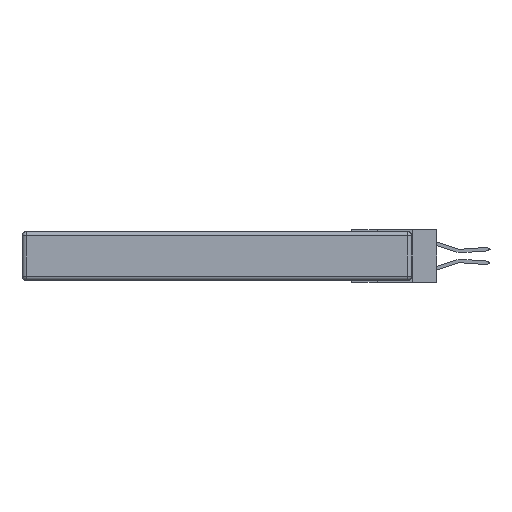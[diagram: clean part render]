
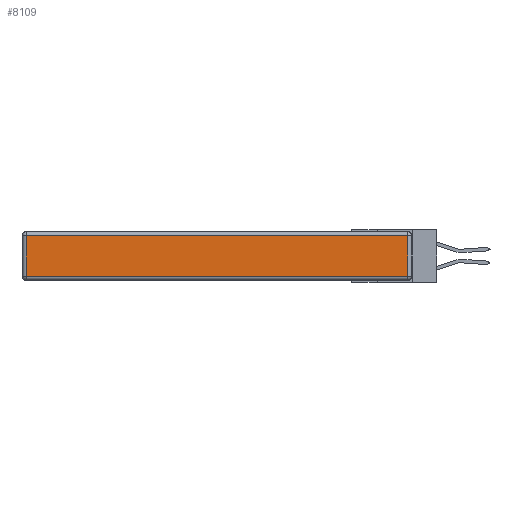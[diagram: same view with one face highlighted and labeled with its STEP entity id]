
A CAD part, left-side view. The second image highlights one B-rep face of the part: STEP entity #8109.
In plain terms, the highlighted planar face has unit normal (-1, 0, 0).
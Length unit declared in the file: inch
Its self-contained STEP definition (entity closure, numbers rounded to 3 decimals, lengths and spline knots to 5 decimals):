
#1151 = VECTOR ( 'NONE', #12823, 39.37008 ) ;
#1198 = DIRECTION ( 'NONE',  ( 0., 0., 1. ) ) ;
#1743 = VECTOR ( 'NONE', #9627, 39.37008 ) ;
#3350 = LINE ( 'NONE', #12667, #1151 ) ;
#3606 = ORIENTED_EDGE ( 'NONE', *, *, #10791, .T. ) ;
#4678 = CARTESIAN_POINT ( 'NONE',  ( 0., 0.03, -0.03 ) ) ;
#4986 = ORIENTED_EDGE ( 'NONE', *, *, #15212, .T. ) ;
#5455 = AXIS2_PLACEMENT_3D ( 'NONE', #11629, #15234, #1198 ) ;
#5585 = CARTESIAN_POINT ( 'NONE',  ( 0., 2.72, -0.03 ) ) ;
#5778 = CARTESIAN_POINT ( 'NONE',  ( 0., 2.72, -0.343 ) ) ;
#5894 = VERTEX_POINT ( 'NONE', #5585 ) ;
#6389 = LINE ( 'NONE', #20187, #1743 ) ;
#7204 = LINE ( 'NONE', #5778, #14309 ) ;
#7402 = VERTEX_POINT ( 'NONE', #13317 ) ;
#8109 = ADVANCED_FACE ( 'NONE', ( #10407 ), #11555, .T. ) ;
#9242 = DIRECTION ( 'NONE',  ( 0., 0., 1. ) ) ;
#9627 = DIRECTION ( 'NONE',  ( 0., -1., 0. ) ) ;
#9665 = EDGE_CURVE ( 'NONE', #5894, #7402, #7204, .T. ) ;
#10407 = FACE_OUTER_BOUND ( 'NONE', #15792, .T. ) ;
#10791 = EDGE_CURVE ( 'NONE', #18504, #5894, #3350, .T. ) ;
#11555 = PLANE ( 'NONE',  #5455 ) ;
#11617 = VERTEX_POINT ( 'NONE', #22510 ) ;
#11629 = CARTESIAN_POINT ( 'NONE',  ( 0., 0., -0.343 ) ) ;
#12127 = VECTOR ( 'NONE', #9242, 39.37008 ) ;
#12667 = CARTESIAN_POINT ( 'NONE',  ( 0., 2.75, -0.03 ) ) ;
#12823 = DIRECTION ( 'NONE',  ( 0., 1., 0. ) ) ;
#13317 = CARTESIAN_POINT ( 'NONE',  ( 0., 2.72, -0.313 ) ) ;
#14309 = VECTOR ( 'NONE', #16009, 39.37008 ) ;
#14340 = LINE ( 'NONE', #17900, #12127 ) ;
#15212 = EDGE_CURVE ( 'NONE', #11617, #18504, #14340, .T. ) ;
#15234 = DIRECTION ( 'NONE',  ( -1., 0., 0. ) ) ;
#15792 = EDGE_LOOP ( 'NONE', ( #19305, #4986, #3606, #20518 ) ) ;
#16009 = DIRECTION ( 'NONE',  ( 0., 0., -1. ) ) ;
#17900 = CARTESIAN_POINT ( 'NONE',  ( 0., 0.03, -0.343 ) ) ;
#18504 = VERTEX_POINT ( 'NONE', #4678 ) ;
#19305 = ORIENTED_EDGE ( 'NONE', *, *, #19415, .T. ) ;
#19415 = EDGE_CURVE ( 'NONE', #7402, #11617, #6389, .T. ) ;
#20187 = CARTESIAN_POINT ( 'NONE',  ( 0., 0., -0.313 ) ) ;
#20518 = ORIENTED_EDGE ( 'NONE', *, *, #9665, .T. ) ;
#22510 = CARTESIAN_POINT ( 'NONE',  ( 0., 0.03, -0.313 ) ) ;
